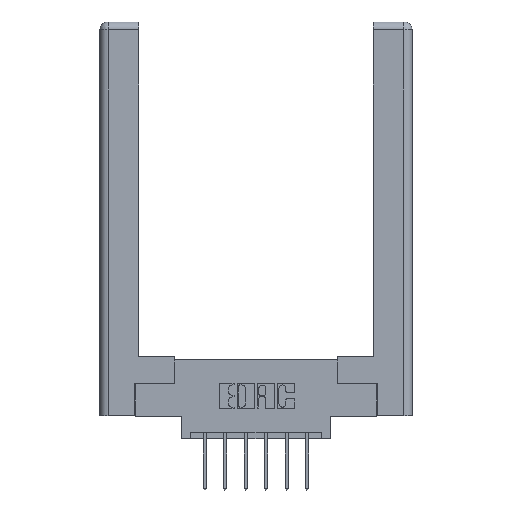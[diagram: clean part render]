
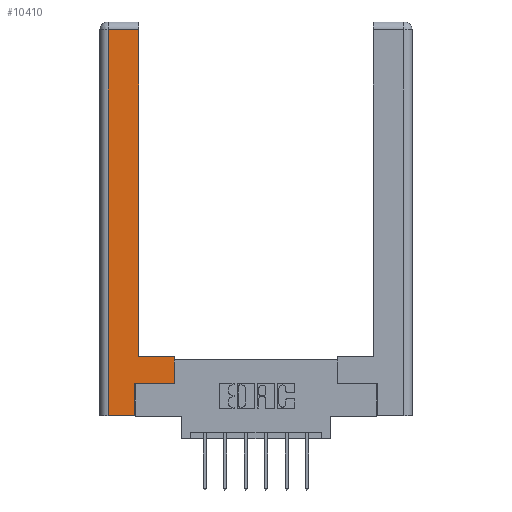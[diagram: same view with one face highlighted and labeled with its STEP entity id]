
A CAD part, top view. The second image highlights one B-rep face of the part: STEP entity #10410.
In plain terms, the highlighted planar face has unit normal (0, 0, 1).
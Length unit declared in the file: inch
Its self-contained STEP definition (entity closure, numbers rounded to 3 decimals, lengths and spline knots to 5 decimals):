
#139 = EDGE_CURVE ( 'NONE', #10107, #11855, #7155, .T. ) ;
#259 = CARTESIAN_POINT ( 'NONE',  ( 0.295, 2.94, 0. ) ) ;
#309 = VECTOR ( 'NONE', #6081, 39.37008 ) ;
#790 = VERTEX_POINT ( 'NONE', #3482 ) ;
#1199 = CARTESIAN_POINT ( 'NONE',  ( 0., 0., 0. ) ) ;
#1206 = LINE ( 'NONE', #8902, #309 ) ;
#1214 = CARTESIAN_POINT ( 'NONE',  ( 0.295, 0.45, 0. ) ) ;
#1399 = VERTEX_POINT ( 'NONE', #9175 ) ;
#1475 = VECTOR ( 'NONE', #4164, 39.37008 ) ;
#1601 = EDGE_CURVE ( 'NONE', #10671, #790, #10779, .T. ) ;
#1610 = EDGE_CURVE ( 'NONE', #6583, #7937, #7417, .T. ) ;
#1765 = LINE ( 'NONE', #3100, #7577 ) ;
#2049 = DIRECTION ( 'NONE',  ( 0., 1., 0. ) ) ;
#2066 = LINE ( 'NONE', #6795, #6135 ) ;
#2069 = EDGE_LOOP ( 'NONE', ( #2544, #6433, #3227, #7065, #3313, #4166, #10752, #2434 ) ) ;
#2125 = AXIS2_PLACEMENT_3D ( 'NONE', #1199, #2151, #8509 ) ;
#2151 = DIRECTION ( 'NONE',  ( 0., 0., -1. ) ) ;
#2312 = CARTESIAN_POINT ( 'NONE',  ( 0.295, 0.45, 0. ) ) ;
#2434 = ORIENTED_EDGE ( 'NONE', *, *, #10498, .T. ) ;
#2544 = ORIENTED_EDGE ( 'NONE', *, *, #139, .T. ) ;
#3100 = CARTESIAN_POINT ( 'NONE',  ( 0.0615, 2.94, 0. ) ) ;
#3227 = ORIENTED_EDGE ( 'NONE', *, *, #8427, .T. ) ;
#3313 = ORIENTED_EDGE ( 'NONE', *, *, #3617, .T. ) ;
#3345 = DIRECTION ( 'NONE',  ( 1., 0., 0. ) ) ;
#3482 = CARTESIAN_POINT ( 'NONE',  ( 0.265, 0., 0. ) ) ;
#3617 = EDGE_CURVE ( 'NONE', #790, #6583, #7969, .T. ) ;
#3661 = VECTOR ( 'NONE', #6090, 39.37008 ) ;
#4164 = DIRECTION ( 'NONE',  ( -1., 0., 0. ) ) ;
#4166 = ORIENTED_EDGE ( 'NONE', *, *, #1610, .T. ) ;
#5191 = CARTESIAN_POINT ( 'NONE',  ( 0.265, 0., 0. ) ) ;
#6079 = DIRECTION ( 'NONE',  ( 1., 0., 0. ) ) ;
#6081 = DIRECTION ( 'NONE',  ( 0., -1., 0. ) ) ;
#6090 = DIRECTION ( 'NONE',  ( 0., 1., 0. ) ) ;
#6135 = VECTOR ( 'NONE', #8690, 39.37008 ) ;
#6433 = ORIENTED_EDGE ( 'NONE', *, *, #7378, .T. ) ;
#6583 = VERTEX_POINT ( 'NONE', #7991 ) ;
#6697 = FACE_OUTER_BOUND ( 'NONE', #2069, .T. ) ;
#6780 = PLANE ( 'NONE',  #2125 ) ;
#6795 = CARTESIAN_POINT ( 'NONE',  ( 0.565, 0.45, 0. ) ) ;
#7065 = ORIENTED_EDGE ( 'NONE', *, *, #1601, .T. ) ;
#7151 = CARTESIAN_POINT ( 'NONE',  ( 0.295, 3., 0. ) ) ;
#7155 = LINE ( 'NONE', #7151, #3661 ) ;
#7378 = EDGE_CURVE ( 'NONE', #11855, #11461, #1765, .T. ) ;
#7417 = LINE ( 'NONE', #8992, #8888 ) ;
#7577 = VECTOR ( 'NONE', #7698, 39.37008 ) ;
#7580 = LINE ( 'NONE', #2312, #1475 ) ;
#7698 = DIRECTION ( 'NONE',  ( -1., 0., 0. ) ) ;
#7937 = VERTEX_POINT ( 'NONE', #11514 ) ;
#7969 = LINE ( 'NONE', #11372, #9161 ) ;
#7991 = CARTESIAN_POINT ( 'NONE',  ( 0.265, 0.245, 0. ) ) ;
#8427 = EDGE_CURVE ( 'NONE', #11461, #10671, #1206, .T. ) ;
#8509 = DIRECTION ( 'NONE',  ( -1., 0., 0. ) ) ;
#8557 = CARTESIAN_POINT ( 'NONE',  ( 0.0615, 2.94, 0. ) ) ;
#8690 = DIRECTION ( 'NONE',  ( 0., 1., 0. ) ) ;
#8888 = VECTOR ( 'NONE', #3345, 39.37008 ) ;
#8902 = CARTESIAN_POINT ( 'NONE',  ( 0.0615, 0., 0. ) ) ;
#8992 = CARTESIAN_POINT ( 'NONE',  ( 0.565, 0.245, 0. ) ) ;
#9161 = VECTOR ( 'NONE', #2049, 39.37008 ) ;
#9175 = CARTESIAN_POINT ( 'NONE',  ( 0.565, 0.45, 0. ) ) ;
#10099 = EDGE_CURVE ( 'NONE', #7937, #1399, #2066, .T. ) ;
#10107 = VERTEX_POINT ( 'NONE', #1214 ) ;
#10410 = ADVANCED_FACE ( 'NONE', ( #6697 ), #6780, .F. ) ;
#10487 = VECTOR ( 'NONE', #6079, 39.37008 ) ;
#10498 = EDGE_CURVE ( 'NONE', #1399, #10107, #7580, .T. ) ;
#10671 = VERTEX_POINT ( 'NONE', #11378 ) ;
#10752 = ORIENTED_EDGE ( 'NONE', *, *, #10099, .T. ) ;
#10779 = LINE ( 'NONE', #5191, #10487 ) ;
#11372 = CARTESIAN_POINT ( 'NONE',  ( 0.265, 0.245, 0. ) ) ;
#11378 = CARTESIAN_POINT ( 'NONE',  ( 0.0615, 0., 0. ) ) ;
#11461 = VERTEX_POINT ( 'NONE', #8557 ) ;
#11514 = CARTESIAN_POINT ( 'NONE',  ( 0.565, 0.245, 0. ) ) ;
#11855 = VERTEX_POINT ( 'NONE', #259 ) ;
